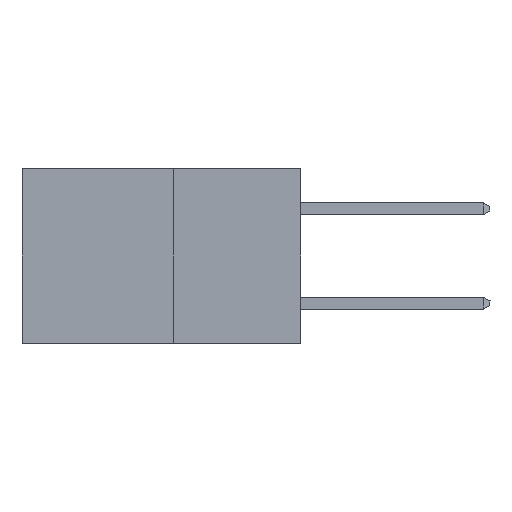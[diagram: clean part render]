
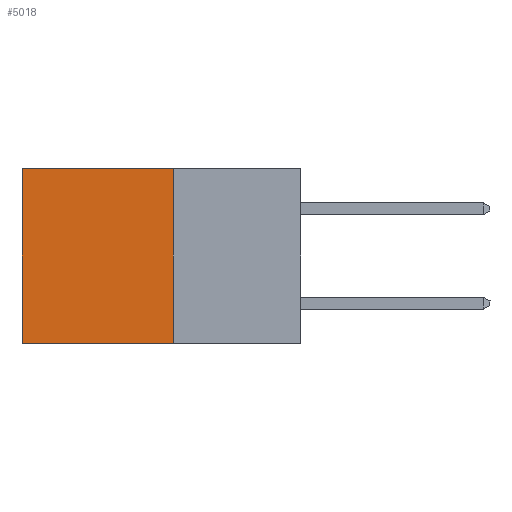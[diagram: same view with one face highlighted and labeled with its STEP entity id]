
A CAD part, left-side view. The second image highlights one B-rep face of the part: STEP entity #5018.
In plain terms, the highlighted planar face has unit normal (-1, 0, 0).
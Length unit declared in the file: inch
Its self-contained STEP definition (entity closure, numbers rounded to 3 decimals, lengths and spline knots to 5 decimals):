
#169 = CARTESIAN_POINT ( 'NONE',  ( 0.277, 0.27, -0.37 ) ) ;
#491 = VERTEX_POINT ( 'NONE', #6465 ) ;
#770 = DIRECTION ( 'NONE',  ( 0., 0., -1. ) ) ;
#882 = VERTEX_POINT ( 'NONE', #7653 ) ;
#1259 = EDGE_CURVE ( 'NONE', #7530, #882, #2349, .T. ) ;
#2155 = EDGE_CURVE ( 'NONE', #491, #7530, #3969, .T. ) ;
#2212 = DIRECTION ( 'NONE',  ( 0., 0., -1. ) ) ;
#2349 = LINE ( 'NONE', #3405, #3902 ) ;
#2406 = EDGE_CURVE ( 'NONE', #4746, #882, #5922, .T. ) ;
#2989 = VECTOR ( 'NONE', #5541, 39.37008 ) ;
#3405 = CARTESIAN_POINT ( 'NONE',  ( 0.277, 0.59, -0.37 ) ) ;
#3607 = CARTESIAN_POINT ( 'NONE',  ( 0.277, 0.27, -0.37 ) ) ;
#3902 = VECTOR ( 'NONE', #2212, 39.37008 ) ;
#3969 = LINE ( 'NONE', #7774, #6582 ) ;
#4746 = VERTEX_POINT ( 'NONE', #169 ) ;
#4968 = CARTESIAN_POINT ( 'NONE',  ( 0.277, 0.59, 0. ) ) ;
#5018 = ADVANCED_FACE ( 'NONE', ( #5442 ), #6969, .F. ) ;
#5128 = ORIENTED_EDGE ( 'NONE', *, *, #2406, .F. ) ;
#5256 = EDGE_CURVE ( 'NONE', #491, #4746, #7222, .T. ) ;
#5299 = ORIENTED_EDGE ( 'NONE', *, *, #2155, .T. ) ;
#5442 = FACE_OUTER_BOUND ( 'NONE', #6782, .T. ) ;
#5541 = DIRECTION ( 'NONE',  ( 0., 1., 0. ) ) ;
#5706 = VECTOR ( 'NONE', #770, 39.37008 ) ;
#5922 = LINE ( 'NONE', #3607, #2989 ) ;
#6092 = CARTESIAN_POINT ( 'NONE',  ( 0.277, 0.27, -0.37 ) ) ;
#6465 = CARTESIAN_POINT ( 'NONE',  ( 0.277, 0.27, 0. ) ) ;
#6575 = ORIENTED_EDGE ( 'NONE', *, *, #1259, .T. ) ;
#6582 = VECTOR ( 'NONE', #6708, 39.37008 ) ;
#6708 = DIRECTION ( 'NONE',  ( 0., 1., 0. ) ) ;
#6782 = EDGE_LOOP ( 'NONE', ( #6575, #5128, #7893, #5299 ) ) ;
#6843 = DIRECTION ( 'NONE',  ( 0., 0., -1. ) ) ;
#6952 = DIRECTION ( 'NONE',  ( 1., 0., 0. ) ) ;
#6969 = PLANE ( 'NONE',  #7895 ) ;
#7222 = LINE ( 'NONE', #6092, #5706 ) ;
#7530 = VERTEX_POINT ( 'NONE', #4968 ) ;
#7653 = CARTESIAN_POINT ( 'NONE',  ( 0.277, 0.59, -0.37 ) ) ;
#7770 = CARTESIAN_POINT ( 'NONE',  ( 0.277, 0.27, -0.37 ) ) ;
#7774 = CARTESIAN_POINT ( 'NONE',  ( 0.277, 0.27, 0. ) ) ;
#7893 = ORIENTED_EDGE ( 'NONE', *, *, #5256, .F. ) ;
#7895 = AXIS2_PLACEMENT_3D ( 'NONE', #7770, #6952, #6843 ) ;
